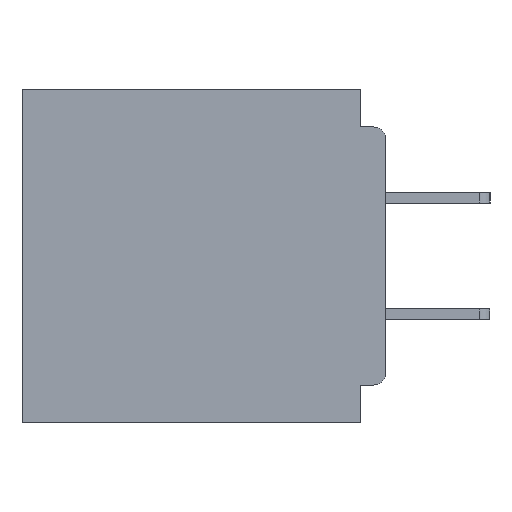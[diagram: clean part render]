
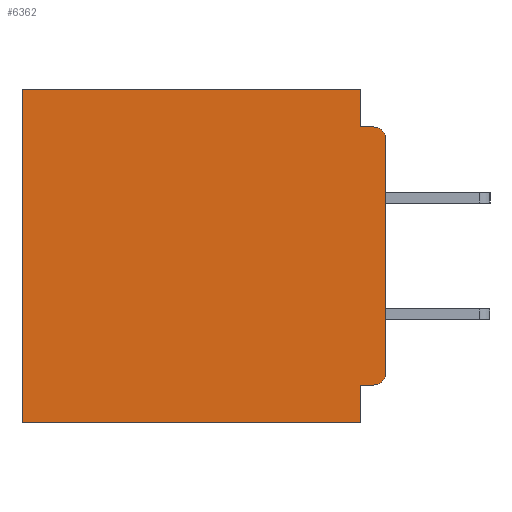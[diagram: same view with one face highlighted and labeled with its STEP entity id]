
A CAD part, left-side view. The second image highlights one B-rep face of the part: STEP entity #6362.
In plain terms, the highlighted planar face has unit normal (-1, 0, 0).
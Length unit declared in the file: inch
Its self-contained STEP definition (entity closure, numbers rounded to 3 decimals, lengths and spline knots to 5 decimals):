
#110 = EDGE_CURVE ( 'NONE', #4259, #45313, #25777, .T. ) ;
#558 = VERTEX_POINT ( 'NONE', #19078 ) ;
#2311 = ORIENTED_EDGE ( 'NONE', *, *, #15767, .T. ) ;
#2965 = CARTESIAN_POINT ( 'NONE',  ( 0.3, 0., -0.045 ) ) ;
#3074 = CARTESIAN_POINT ( 'NONE',  ( 0.3, 0.437, -0.4 ) ) ;
#4259 = VERTEX_POINT ( 'NONE', #35437 ) ;
#4574 = EDGE_CURVE ( 'NONE', #558, #24245, #44705, .T. ) ;
#4717 = CIRCLE ( 'NONE', #19558, 0.015 ) ;
#5353 = ORIENTED_EDGE ( 'NONE', *, *, #4574, .F. ) ;
#5498 = DIRECTION ( 'NONE',  ( 0., 0., -1. ) ) ;
#6039 = ORIENTED_EDGE ( 'NONE', *, *, #48307, .F. ) ;
#6268 = VECTOR ( 'NONE', #46240, 39.37008 ) ;
#6362 = ADVANCED_FACE ( 'NONE', ( #15982 ), #39602, .F. ) ;
#6440 = VECTOR ( 'NONE', #18098, 39.37008 ) ;
#6752 = CARTESIAN_POINT ( 'NONE',  ( 0.3, 0.031, 0. ) ) ;
#7357 = LINE ( 'NONE', #33194, #45920 ) ;
#7363 = ORIENTED_EDGE ( 'NONE', *, *, #18328, .T. ) ;
#9310 = CARTESIAN_POINT ( 'NONE',  ( 0.3, 0., -0.4 ) ) ;
#9472 = DIRECTION ( 'NONE',  ( 0., 1., 0. ) ) ;
#10889 = VERTEX_POINT ( 'NONE', #25509 ) ;
#11695 = VECTOR ( 'NONE', #20216, 39.37008 ) ;
#12587 = LINE ( 'NONE', #18621, #31273 ) ;
#12977 = LINE ( 'NONE', #24189, #30478 ) ;
#13183 = ORIENTED_EDGE ( 'NONE', *, *, #110, .T. ) ;
#13396 = ORIENTED_EDGE ( 'NONE', *, *, #38581, .F. ) ;
#14817 = VERTEX_POINT ( 'NONE', #27021 ) ;
#14947 = ORIENTED_EDGE ( 'NONE', *, *, #30869, .F. ) ;
#15608 = EDGE_CURVE ( 'NONE', #4259, #37804, #12977, .T. ) ;
#15767 = EDGE_CURVE ( 'NONE', #14817, #37804, #4717, .T. ) ;
#15982 = FACE_OUTER_BOUND ( 'NONE', #29125, .T. ) ;
#16447 = EDGE_CURVE ( 'NONE', #42738, #24245, #30381, .T. ) ;
#17189 = CARTESIAN_POINT ( 'NONE',  ( 0.3, 0., -0.34 ) ) ;
#17287 = CARTESIAN_POINT ( 'NONE',  ( 0.3, 0., -0.4 ) ) ;
#17659 = DIRECTION ( 'NONE',  ( -1., 0., 0. ) ) ;
#18070 = VERTEX_POINT ( 'NONE', #40907 ) ;
#18098 = DIRECTION ( 'NONE',  ( 0., -1., 0. ) ) ;
#18258 = VERTEX_POINT ( 'NONE', #30781 ) ;
#18328 = EDGE_CURVE ( 'NONE', #18070, #42738, #36105, .T. ) ;
#18621 = CARTESIAN_POINT ( 'NONE',  ( 0.3, 0., -0.355 ) ) ;
#19078 = CARTESIAN_POINT ( 'NONE',  ( 0.3, 0.031, -0.4 ) ) ;
#19423 = ORIENTED_EDGE ( 'NONE', *, *, #41587, .F. ) ;
#19558 = AXIS2_PLACEMENT_3D ( 'NONE', #39984, #17659, #43735 ) ;
#20216 = DIRECTION ( 'NONE',  ( 0., 0., -1. ) ) ;
#21052 = DIRECTION ( 'NONE',  ( 1., 0., 0. ) ) ;
#21792 = VECTOR ( 'NONE', #25458, 39.37008 ) ;
#22374 = CARTESIAN_POINT ( 'NONE',  ( 0.3, 0.015, -0.045 ) ) ;
#24189 = CARTESIAN_POINT ( 'NONE',  ( 0.3, 0., -0.4 ) ) ;
#24245 = VERTEX_POINT ( 'NONE', #3074 ) ;
#25458 = DIRECTION ( 'NONE',  ( 0., 0., -1. ) ) ;
#25509 = CARTESIAN_POINT ( 'NONE',  ( 0.3, 0.031, -0.355 ) ) ;
#25777 = CIRCLE ( 'NONE', #33596, 0.015 ) ;
#26085 = VECTOR ( 'NONE', #9472, 39.37008 ) ;
#27021 = CARTESIAN_POINT ( 'NONE',  ( 0.3, 0.015, -0.355 ) ) ;
#29125 = EDGE_LOOP ( 'NONE', ( #35522, #13183, #6039, #13396, #7363, #47987, #5353, #14947, #19423, #2311 ) ) ;
#30381 = LINE ( 'NONE', #38767, #11695 ) ;
#30478 = VECTOR ( 'NONE', #5498, 39.37008 ) ;
#30781 = CARTESIAN_POINT ( 'NONE',  ( 0.3, 0.031, -0.045 ) ) ;
#30869 = EDGE_CURVE ( 'NONE', #10889, #558, #7357, .T. ) ;
#31273 = VECTOR ( 'NONE', #40929, 39.37008 ) ;
#33194 = CARTESIAN_POINT ( 'NONE',  ( 0.3, 0.031, -0.4 ) ) ;
#33596 = AXIS2_PLACEMENT_3D ( 'NONE', #47437, #34044, #46701 ) ;
#34044 = DIRECTION ( 'NONE',  ( -1., 0., 0. ) ) ;
#35437 = CARTESIAN_POINT ( 'NONE',  ( 0.3, 0., -0.06 ) ) ;
#35522 = ORIENTED_EDGE ( 'NONE', *, *, #15608, .F. ) ;
#36105 = LINE ( 'NONE', #42528, #6268 ) ;
#36581 = AXIS2_PLACEMENT_3D ( 'NONE', #17287, #21052, #47086 ) ;
#37804 = VERTEX_POINT ( 'NONE', #17189 ) ;
#38581 = EDGE_CURVE ( 'NONE', #18070, #18258, #41607, .T. ) ;
#38767 = CARTESIAN_POINT ( 'NONE',  ( 0.3, 0.437, -0.4 ) ) ;
#39602 = PLANE ( 'NONE',  #36581 ) ;
#39984 = CARTESIAN_POINT ( 'NONE',  ( 0.3, 0.015, -0.34 ) ) ;
#40907 = CARTESIAN_POINT ( 'NONE',  ( 0.3, 0.031, 0. ) ) ;
#40929 = DIRECTION ( 'NONE',  ( 0., 1., 0. ) ) ;
#41587 = EDGE_CURVE ( 'NONE', #14817, #10889, #12587, .T. ) ;
#41607 = LINE ( 'NONE', #6752, #21792 ) ;
#42528 = CARTESIAN_POINT ( 'NONE',  ( 0.3, 0., 0. ) ) ;
#42738 = VERTEX_POINT ( 'NONE', #43337 ) ;
#43337 = CARTESIAN_POINT ( 'NONE',  ( 0.3, 0.437, 0. ) ) ;
#43735 = DIRECTION ( 'NONE',  ( 0., 0., -1. ) ) ;
#44286 = DIRECTION ( 'NONE',  ( 0., 0., -1. ) ) ;
#44705 = LINE ( 'NONE', #9310, #26085 ) ;
#44994 = LINE ( 'NONE', #2965, #6440 ) ;
#45313 = VERTEX_POINT ( 'NONE', #22374 ) ;
#45920 = VECTOR ( 'NONE', #44286, 39.37008 ) ;
#46240 = DIRECTION ( 'NONE',  ( 0., 1., 0. ) ) ;
#46701 = DIRECTION ( 'NONE',  ( 0., 0., -1. ) ) ;
#47086 = DIRECTION ( 'NONE',  ( 0., 0., -1. ) ) ;
#47437 = CARTESIAN_POINT ( 'NONE',  ( 0.3, 0.015, -0.06 ) ) ;
#47987 = ORIENTED_EDGE ( 'NONE', *, *, #16447, .T. ) ;
#48307 = EDGE_CURVE ( 'NONE', #18258, #45313, #44994, .T. ) ;
